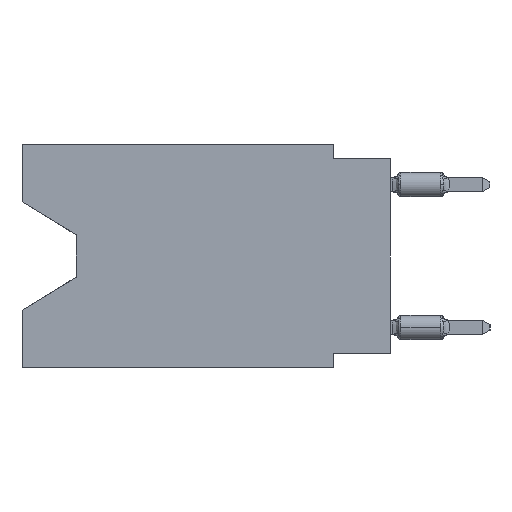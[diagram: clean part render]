
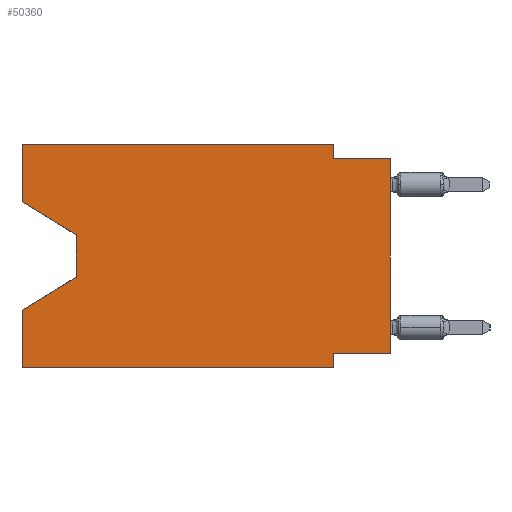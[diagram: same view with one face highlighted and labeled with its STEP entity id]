
A CAD part, left-side view. The second image highlights one B-rep face of the part: STEP entity #50360.
In plain terms, the highlighted planar face has unit normal (-1, 0, 0).
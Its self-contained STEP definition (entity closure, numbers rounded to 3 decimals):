
#366 = EDGE_CURVE ( 'NONE', #27638, #48048, #43433, .T. ) ;
#395 = DIRECTION ( 'NONE',  ( 0., 0., -1. ) ) ;
#990 = VERTEX_POINT ( 'NONE', #49012 ) ;
#1702 = CARTESIAN_POINT ( 'NONE',  ( 0., 2.54, -9.906 ) ) ;
#3009 = DIRECTION ( 'NONE',  ( 0., -1., 0. ) ) ;
#3631 = CARTESIAN_POINT ( 'NONE',  ( 0., 0., 0. ) ) ;
#4603 = ORIENTED_EDGE ( 'NONE', *, *, #45052, .T. ) ;
#5527 = DIRECTION ( 'NONE',  ( 0., 1., 0. ) ) ;
#5653 = LINE ( 'NONE', #34690, #32305 ) ;
#5956 = EDGE_LOOP ( 'NONE', ( #18274, #12540, #4603, #33024, #27982, #36836, #49328, #51446, #46434, #51716, #46038, #30994 ) ) ;
#6260 = CARTESIAN_POINT ( 'NONE',  ( 0., 13.97, -4.013 ) ) ;
#6533 = LINE ( 'NONE', #39912, #35962 ) ;
#7099 = LINE ( 'NONE', #36126, #41897 ) ;
#7706 = CARTESIAN_POINT ( 'NONE',  ( 0., 13.97, -5.893 ) ) ;
#8237 = CARTESIAN_POINT ( 'NONE',  ( 0., 2.54, 0. ) ) ;
#8280 = VERTEX_POINT ( 'NONE', #31680 ) ;
#8831 = EDGE_CURVE ( 'NONE', #18729, #990, #50558, .T. ) ;
#9342 = VECTOR ( 'NONE', #26986, 1000. ) ;
#10386 = EDGE_CURVE ( 'NONE', #25895, #33167, #49784, .T. ) ;
#11005 = DIRECTION ( 'NONE',  ( 0., 0., -1. ) ) ;
#12421 = DIRECTION ( 'NONE',  ( 0., 0., -1. ) ) ;
#12540 = ORIENTED_EDGE ( 'NONE', *, *, #366, .T. ) ;
#12641 = CARTESIAN_POINT ( 'NONE',  ( 0., 2.54, -0.635 ) ) ;
#12692 = CARTESIAN_POINT ( 'NONE',  ( 0., 16.383, 0. ) ) ;
#13520 = VECTOR ( 'NONE', #24251, 1000. ) ;
#13685 = CARTESIAN_POINT ( 'NONE',  ( 0., 16.383, 0. ) ) ;
#15077 = VECTOR ( 'NONE', #35030, 1000. ) ;
#15335 = CARTESIAN_POINT ( 'NONE',  ( 0., 2.54, -9.906 ) ) ;
#17854 = VECTOR ( 'NONE', #48157, 1000. ) ;
#18274 = ORIENTED_EDGE ( 'NONE', *, *, #35038, .T. ) ;
#18529 = CARTESIAN_POINT ( 'NONE',  ( 0., 0., -9.271 ) ) ;
#18729 = VERTEX_POINT ( 'NONE', #27725 ) ;
#19749 = CARTESIAN_POINT ( 'NONE',  ( 0., 16.383, 0. ) ) ;
#20485 = VECTOR ( 'NONE', #11005, 1000. ) ;
#20819 = FACE_OUTER_BOUND ( 'NONE', #5956, .T. ) ;
#20881 = CARTESIAN_POINT ( 'NONE',  ( 0., 13.97, -5.893 ) ) ;
#21063 = VERTEX_POINT ( 'NONE', #1702 ) ;
#21266 = VECTOR ( 'NONE', #48218, 1000. ) ;
#23329 = AXIS2_PLACEMENT_3D ( 'NONE', #19749, #41193, #12421 ) ;
#23746 = VERTEX_POINT ( 'NONE', #12692 ) ;
#24226 = VECTOR ( 'NONE', #5527, 1000. ) ;
#24251 = DIRECTION ( 'NONE',  ( 0., 0.855, -0.519 ) ) ;
#24562 = VERTEX_POINT ( 'NONE', #44605 ) ;
#24816 = CARTESIAN_POINT ( 'NONE',  ( 0., 2.54, 0. ) ) ;
#24958 = DIRECTION ( 'NONE',  ( 0., -1., 0. ) ) ;
#25895 = VERTEX_POINT ( 'NONE', #8237 ) ;
#25902 = LINE ( 'NONE', #13685, #9342 ) ;
#26986 = DIRECTION ( 'NONE',  ( 0., 0., 1. ) ) ;
#27638 = VERTEX_POINT ( 'NONE', #28790 ) ;
#27725 = CARTESIAN_POINT ( 'NONE',  ( 0., 0., -9.271 ) ) ;
#27982 = ORIENTED_EDGE ( 'NONE', *, *, #44574, .T. ) ;
#28143 = CARTESIAN_POINT ( 'NONE',  ( 0., 16.383, -9.906 ) ) ;
#28337 = LINE ( 'NONE', #7706, #13520 ) ;
#28790 = CARTESIAN_POINT ( 'NONE',  ( 0., 13.97, -4.013 ) ) ;
#29578 = LINE ( 'NONE', #38260, #48278 ) ;
#30994 = ORIENTED_EDGE ( 'NONE', *, *, #37046, .F. ) ;
#31680 = CARTESIAN_POINT ( 'NONE',  ( 0., 16.383, -2.546 ) ) ;
#32233 = VERTEX_POINT ( 'NONE', #53220 ) ;
#32305 = VECTOR ( 'NONE', #46886, 1000. ) ;
#33024 = ORIENTED_EDGE ( 'NONE', *, *, #41031, .F. ) ;
#33118 = CARTESIAN_POINT ( 'NONE',  ( 0., 16.383, -9.906 ) ) ;
#33167 = VERTEX_POINT ( 'NONE', #12641 ) ;
#34690 = CARTESIAN_POINT ( 'NONE',  ( 0., 16.383, -2.546 ) ) ;
#35030 = DIRECTION ( 'NONE',  ( 0., 0., -1. ) ) ;
#35038 = EDGE_CURVE ( 'NONE', #8280, #27638, #5653, .T. ) ;
#35703 = LINE ( 'NONE', #3631, #17854 ) ;
#35962 = VECTOR ( 'NONE', #51572, 1000. ) ;
#36126 = CARTESIAN_POINT ( 'NONE',  ( 0., 16.383, 0. ) ) ;
#36836 = ORIENTED_EDGE ( 'NONE', *, *, #38068, .F. ) ;
#37046 = EDGE_CURVE ( 'NONE', #8280, #23746, #6533, .T. ) ;
#38068 = EDGE_CURVE ( 'NONE', #990, #21063, #48174, .T. ) ;
#38260 = CARTESIAN_POINT ( 'NONE',  ( 0., 0., -0.635 ) ) ;
#39912 = CARTESIAN_POINT ( 'NONE',  ( 0., 16.383, 0. ) ) ;
#40067 = EDGE_CURVE ( 'NONE', #33167, #24562, #29578, .T. ) ;
#41031 = EDGE_CURVE ( 'NONE', #49917, #32233, #25902, .T. ) ;
#41193 = DIRECTION ( 'NONE',  ( 1., 0., 0. ) ) ;
#41531 = EDGE_CURVE ( 'NONE', #23746, #25895, #7099, .T. ) ;
#41897 = VECTOR ( 'NONE', #3009, 1000. ) ;
#43433 = LINE ( 'NONE', #6260, #15077 ) ;
#44574 = EDGE_CURVE ( 'NONE', #49917, #21063, #44675, .T. ) ;
#44605 = CARTESIAN_POINT ( 'NONE',  ( 0., 0., -0.635 ) ) ;
#44675 = LINE ( 'NONE', #28143, #21266 ) ;
#45052 = EDGE_CURVE ( 'NONE', #48048, #32233, #28337, .T. ) ;
#45068 = EDGE_CURVE ( 'NONE', #18729, #24562, #35703, .T. ) ;
#46038 = ORIENTED_EDGE ( 'NONE', *, *, #41531, .F. ) ;
#46434 = ORIENTED_EDGE ( 'NONE', *, *, #40067, .F. ) ;
#46886 = DIRECTION ( 'NONE',  ( 0., -0.855, -0.519 ) ) ;
#48048 = VERTEX_POINT ( 'NONE', #20881 ) ;
#48157 = DIRECTION ( 'NONE',  ( 0., 0., 1. ) ) ;
#48174 = LINE ( 'NONE', #15335, #20485 ) ;
#48218 = DIRECTION ( 'NONE',  ( 0., -1., 0. ) ) ;
#48278 = VECTOR ( 'NONE', #24958, 1000. ) ;
#49012 = CARTESIAN_POINT ( 'NONE',  ( 0., 2.54, -9.271 ) ) ;
#49328 = ORIENTED_EDGE ( 'NONE', *, *, #8831, .F. ) ;
#49599 = PLANE ( 'NONE',  #23329 ) ;
#49784 = LINE ( 'NONE', #24816, #52886 ) ;
#49917 = VERTEX_POINT ( 'NONE', #33118 ) ;
#50360 = ADVANCED_FACE ( 'NONE', ( #20819 ), #49599, .F. ) ;
#50558 = LINE ( 'NONE', #18529, #24226 ) ;
#51446 = ORIENTED_EDGE ( 'NONE', *, *, #45068, .T. ) ;
#51572 = DIRECTION ( 'NONE',  ( 0., 0., 1. ) ) ;
#51716 = ORIENTED_EDGE ( 'NONE', *, *, #10386, .F. ) ;
#52886 = VECTOR ( 'NONE', #395, 1000. ) ;
#53220 = CARTESIAN_POINT ( 'NONE',  ( 0., 16.383, -7.36 ) ) ;
